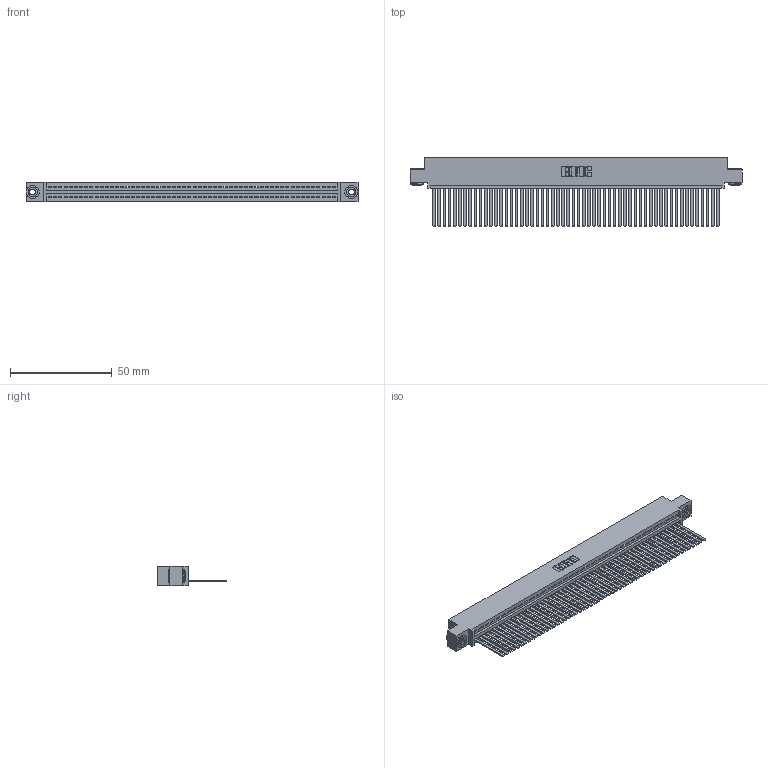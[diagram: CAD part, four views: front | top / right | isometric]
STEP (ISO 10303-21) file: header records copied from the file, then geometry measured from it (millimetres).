
FILE_DESCRIPTION (( 'STEP AP203' ), '1' );
FILE_NAME ('345-056-544-403.STEP', '2018-09-25T19:31:34', ( '' ), ( '' ), 'SwSTEP 2.0', 'SolidWorks 2016', '' );
FILE_SCHEMA (( 'CONFIG_CONTROL_DESIGN' ));
Length unit declared in the file: inch
Products named in the file (4): 345 Part_0.110 Offset - 0.156 Dia-TH; 345-056-544-403; 345-250-002_345-250-002-102; 345-292-001_345-293-144
Assembly tree (59 placements, depth 2):
  345-056-544-403
    345 Part_0.110 Offset - 0.156 Dia-TH
    345-292-001_345-293-144  x56
    345-250-002_345-250-002-102  x2
Bounding box: 163.45 x 33.96 x 9.4 mm (x, y, z)
Volume: 16233.8 mm3; surface area: 24006.9 mm2
Topology: 59 solids, 59 shells, 3080 faces, 9277 edges, 6106 vertices
Faces by surface type: plane 2110, cylinder 962, cone 8
Entity records: 40860 total; most frequent: CARTESIAN_POINT 7055, ORIENTED_EDGE 7038, DIRECTION 6169, EDGE_CURVE 3519, LINE 3143, VECTOR 3143, VERTEX_POINT 2342, AXIS2_PLACEMENT_3D 1513
